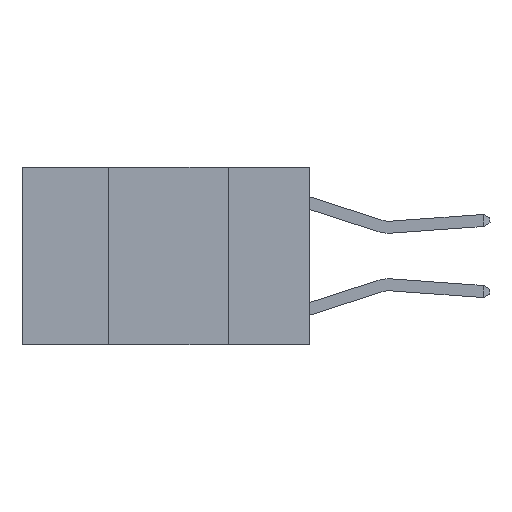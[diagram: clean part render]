
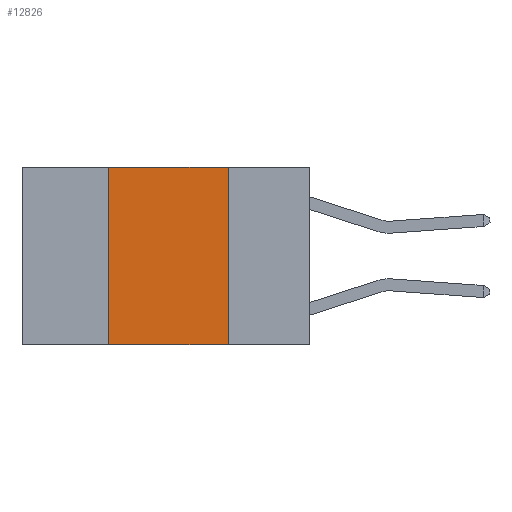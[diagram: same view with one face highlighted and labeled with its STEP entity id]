
A CAD part, left-side view. The second image highlights one B-rep face of the part: STEP entity #12826.
In plain terms, the highlighted planar face has unit normal (-1, 0, 0).
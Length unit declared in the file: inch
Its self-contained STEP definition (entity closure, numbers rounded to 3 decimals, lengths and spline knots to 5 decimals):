
#545 = DIRECTION ( 'NONE',  ( 0., -1., 0. ) ) ;
#1222 = VECTOR ( 'NONE', #7375, 39.37008 ) ;
#2897 = CARTESIAN_POINT ( 'NONE',  ( 0., 0.42, -0.37 ) ) ;
#4035 = AXIS2_PLACEMENT_3D ( 'NONE', #5463, #27197, #14266 ) ;
#5463 = CARTESIAN_POINT ( 'NONE',  ( 0., 0.6, 0. ) ) ;
#6281 = LINE ( 'NONE', #24106, #11432 ) ;
#7375 = DIRECTION ( 'NONE',  ( 0., -1., 0. ) ) ;
#7729 = ORIENTED_EDGE ( 'NONE', *, *, #15433, .F. ) ;
#7794 = VERTEX_POINT ( 'NONE', #22178 ) ;
#7827 = LINE ( 'NONE', #22445, #25180 ) ;
#9558 = DIRECTION ( 'NONE',  ( 0., 0., 1. ) ) ;
#10328 = VERTEX_POINT ( 'NONE', #14982 ) ;
#10529 = EDGE_LOOP ( 'NONE', ( #7729, #22092, #14084, #20258 ) ) ;
#11432 = VECTOR ( 'NONE', #13284, 39.37008 ) ;
#11574 = CARTESIAN_POINT ( 'NONE',  ( 0., 0.42, 0. ) ) ;
#12675 = EDGE_CURVE ( 'NONE', #7794, #10328, #7827, .T. ) ;
#12826 = ADVANCED_FACE ( 'NONE', ( #27474 ), #24979, .F. ) ;
#13284 = DIRECTION ( 'NONE',  ( 0., 0., -1. ) ) ;
#14084 = ORIENTED_EDGE ( 'NONE', *, *, #18381, .F. ) ;
#14266 = DIRECTION ( 'NONE',  ( 0., 0., -1. ) ) ;
#14982 = CARTESIAN_POINT ( 'NONE',  ( 0., 0.17, 0. ) ) ;
#15433 = EDGE_CURVE ( 'NONE', #10328, #21285, #6281, .T. ) ;
#16871 = LINE ( 'NONE', #11574, #27611 ) ;
#17343 = LINE ( 'NONE', #26831, #1222 ) ;
#18381 = EDGE_CURVE ( 'NONE', #22976, #7794, #16871, .T. ) ;
#20258 = ORIENTED_EDGE ( 'NONE', *, *, #22705, .T. ) ;
#21285 = VERTEX_POINT ( 'NONE', #24761 ) ;
#22092 = ORIENTED_EDGE ( 'NONE', *, *, #12675, .F. ) ;
#22178 = CARTESIAN_POINT ( 'NONE',  ( 0., 0.42, 0. ) ) ;
#22445 = CARTESIAN_POINT ( 'NONE',  ( 0., 0.6, 0. ) ) ;
#22705 = EDGE_CURVE ( 'NONE', #22976, #21285, #17343, .T. ) ;
#22976 = VERTEX_POINT ( 'NONE', #2897 ) ;
#24106 = CARTESIAN_POINT ( 'NONE',  ( 0., 0.17, 0. ) ) ;
#24761 = CARTESIAN_POINT ( 'NONE',  ( 0., 0.17, -0.37 ) ) ;
#24979 = PLANE ( 'NONE',  #4035 ) ;
#25180 = VECTOR ( 'NONE', #545, 39.37008 ) ;
#26831 = CARTESIAN_POINT ( 'NONE',  ( 0., 0.6, -0.37 ) ) ;
#27197 = DIRECTION ( 'NONE',  ( 1., 0., 0. ) ) ;
#27474 = FACE_OUTER_BOUND ( 'NONE', #10529, .T. ) ;
#27611 = VECTOR ( 'NONE', #9558, 39.37008 ) ;
